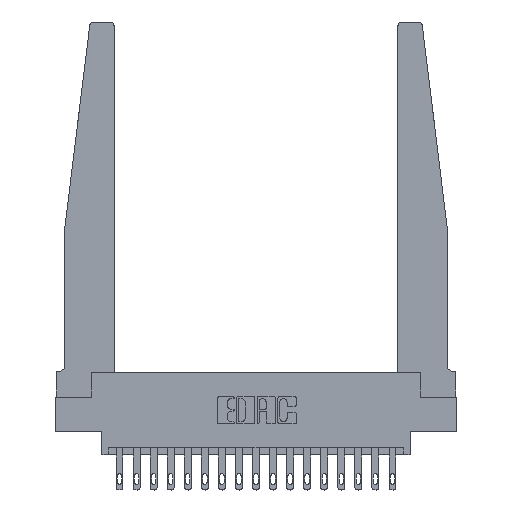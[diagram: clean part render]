
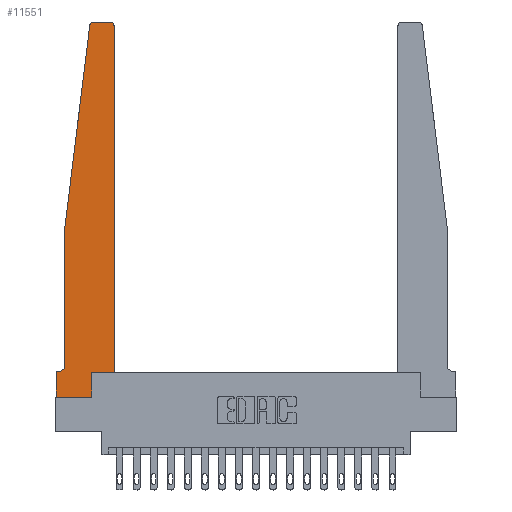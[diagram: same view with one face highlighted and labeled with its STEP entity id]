
A CAD part, top view. The second image highlights one B-rep face of the part: STEP entity #11551.
In plain terms, the highlighted planar face has unit normal (0, 0, 1).
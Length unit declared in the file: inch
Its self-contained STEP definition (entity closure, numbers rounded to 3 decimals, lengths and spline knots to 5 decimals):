
#142 = CARTESIAN_POINT ( 'NONE',  ( 0.425, 0.18, 0.37 ) ) ;
#512 = DIRECTION ( 'NONE',  ( 0., 0., 1. ) ) ;
#813 = AXIS2_PLACEMENT_3D ( 'NONE', #14838, #11664, #16329 ) ;
#840 = VECTOR ( 'NONE', #6981, 39.37008 ) ;
#849 = ORIENTED_EDGE ( 'NONE', *, *, #18544, .T. ) ;
#868 = VECTOR ( 'NONE', #9005, 39.37008 ) ;
#875 = CARTESIAN_POINT ( 'NONE',  ( 0., 0., 0.37 ) ) ;
#973 = CARTESIAN_POINT ( 'NONE',  ( 0.015, 0.2375, 0.37 ) ) ;
#1383 = ORIENTED_EDGE ( 'NONE', *, *, #11961, .T. ) ;
#1763 = VECTOR ( 'NONE', #14503, 39.37008 ) ;
#1956 = CARTESIAN_POINT ( 'NONE',  ( 0.065, 0.2375, 0.37 ) ) ;
#2150 = EDGE_CURVE ( 'NONE', #18866, #17436, #12518, .T. ) ;
#2842 = LINE ( 'NONE', #142, #8823 ) ;
#2949 = ORIENTED_EDGE ( 'NONE', *, *, #14845, .T. ) ;
#3259 = VECTOR ( 'NONE', #5181, 39.37008 ) ;
#3283 = VERTEX_POINT ( 'NONE', #7227 ) ;
#3580 = DIRECTION ( 'NONE',  ( -1., 0., 0. ) ) ;
#3769 = CIRCLE ( 'NONE', #6992, 0.05 ) ;
#3858 = LINE ( 'NONE', #875, #840 ) ;
#3860 = DIRECTION ( 'NONE',  ( 0., -1., 0. ) ) ;
#3970 = VECTOR ( 'NONE', #3860, 39.37008 ) ;
#3993 = EDGE_CURVE ( 'NONE', #12755, #3283, #17140, .T. ) ;
#4364 = VERTEX_POINT ( 'NONE', #14314 ) ;
#4394 = VERTEX_POINT ( 'NONE', #17504 ) ;
#4511 = CARTESIAN_POINT ( 'NONE',  ( 0.2605, 0.18, 0.37 ) ) ;
#4976 = LINE ( 'NONE', #9862, #17024 ) ;
#5012 = CARTESIAN_POINT ( 'NONE',  ( 0., 0.1875, 0.37 ) ) ;
#5181 = DIRECTION ( 'NONE',  ( -1., 0., 0. ) ) ;
#5279 = CIRCLE ( 'NONE', #813, 0.03 ) ;
#5324 = LINE ( 'NONE', #12832, #1763 ) ;
#5334 = AXIS2_PLACEMENT_3D ( 'NONE', #7943, #6639, #14203 ) ;
#5372 = LINE ( 'NONE', #11483, #3970 ) ;
#6398 = VECTOR ( 'NONE', #7916, 39.37008 ) ;
#6484 = ORIENTED_EDGE ( 'NONE', *, *, #13730, .T. ) ;
#6507 = ORIENTED_EDGE ( 'NONE', *, *, #13590, .T. ) ;
#6639 = DIRECTION ( 'NONE',  ( 0., 0., 1. ) ) ;
#6855 = VECTOR ( 'NONE', #16029, 39.37008 ) ;
#6981 = DIRECTION ( 'NONE',  ( 0., -1., 0. ) ) ;
#6992 = AXIS2_PLACEMENT_3D ( 'NONE', #973, #11200, #3580 ) ;
#6995 = CARTESIAN_POINT ( 'NONE',  ( 0.425, 0.18, 0.37 ) ) ;
#7227 = CARTESIAN_POINT ( 'NONE',  ( 0.27653, 2.75, 0.37 ) ) ;
#7452 = CARTESIAN_POINT ( 'NONE',  ( 0.2605, 0., 0.37 ) ) ;
#7617 = ORIENTED_EDGE ( 'NONE', *, *, #2150, .T. ) ;
#7916 = DIRECTION ( 'NONE',  ( 0., 1., 0. ) ) ;
#7943 = CARTESIAN_POINT ( 'NONE',  ( 0.27653, 2.72, 0.37 ) ) ;
#8084 = DIRECTION ( 'NONE',  ( 1., 0., 0. ) ) ;
#8559 = VERTEX_POINT ( 'NONE', #5012 ) ;
#8823 = VECTOR ( 'NONE', #16498, 39.37008 ) ;
#9005 = DIRECTION ( 'NONE',  ( -0.122, -0.992, 0. ) ) ;
#9197 = VERTEX_POINT ( 'NONE', #6995 ) ;
#9204 = CARTESIAN_POINT ( 'NONE',  ( 0.425, 2.72, 0.37 ) ) ;
#9537 = EDGE_LOOP ( 'NONE', ( #12274, #9996, #849, #6484, #1383, #16868, #16133, #2949, #7617, #6507, #15865, #16618 ) ) ;
#9605 = VERTEX_POINT ( 'NONE', #1956 ) ;
#9862 = CARTESIAN_POINT ( 'NONE',  ( 0.425, 0.18, 0.37 ) ) ;
#9996 = ORIENTED_EDGE ( 'NONE', *, *, #18228, .T. ) ;
#10084 = CARTESIAN_POINT ( 'NONE',  ( 0.015, 0.1875, 0.37 ) ) ;
#11200 = DIRECTION ( 'NONE',  ( 0., 0., -1. ) ) ;
#11419 = FACE_OUTER_BOUND ( 'NONE', #9537, .T. ) ;
#11473 = CARTESIAN_POINT ( 'NONE',  ( 0., 0., 0.37 ) ) ;
#11483 = CARTESIAN_POINT ( 'NONE',  ( 0.065, 1.25, 0.37 ) ) ;
#11551 = ADVANCED_FACE ( 'NONE', ( #11419 ), #18980, .T. ) ;
#11660 = LINE ( 'NONE', #11473, #6855 ) ;
#11664 = DIRECTION ( 'NONE',  ( 0., 0., 1. ) ) ;
#11961 = EDGE_CURVE ( 'NONE', #9605, #14570, #3769, .T. ) ;
#12274 = ORIENTED_EDGE ( 'NONE', *, *, #3993, .T. ) ;
#12518 = LINE ( 'NONE', #4511, #6398 ) ;
#12594 = CARTESIAN_POINT ( 'NONE',  ( 0.25, 2.75, 0.37 ) ) ;
#12755 = VERTEX_POINT ( 'NONE', #16577 ) ;
#12832 = CARTESIAN_POINT ( 'NONE',  ( 0.065, 0.1875, 0.37 ) ) ;
#13590 = EDGE_CURVE ( 'NONE', #17436, #9197, #4976, .T. ) ;
#13730 = EDGE_CURVE ( 'NONE', #4364, #9605, #5372, .T. ) ;
#14032 = EDGE_CURVE ( 'NONE', #14570, #8559, #5324, .T. ) ;
#14203 = DIRECTION ( 'NONE',  ( 1., 0., 0. ) ) ;
#14295 = VERTEX_POINT ( 'NONE', #9204 ) ;
#14314 = CARTESIAN_POINT ( 'NONE',  ( 0.065, 1.25, 0.37 ) ) ;
#14394 = CARTESIAN_POINT ( 'NONE',  ( 0., 0.1875, 0.37 ) ) ;
#14503 = DIRECTION ( 'NONE',  ( -1., 0., 0. ) ) ;
#14570 = VERTEX_POINT ( 'NONE', #10084 ) ;
#14838 = CARTESIAN_POINT ( 'NONE',  ( 0.395, 2.72, 0.37 ) ) ;
#14845 = EDGE_CURVE ( 'NONE', #15749, #18866, #11660, .T. ) ;
#15749 = VERTEX_POINT ( 'NONE', #16350 ) ;
#15865 = ORIENTED_EDGE ( 'NONE', *, *, #18075, .T. ) ;
#16029 = DIRECTION ( 'NONE',  ( 1., 0., 0. ) ) ;
#16133 = ORIENTED_EDGE ( 'NONE', *, *, #17519, .T. ) ;
#16172 = EDGE_CURVE ( 'NONE', #14295, #12755, #5279, .T. ) ;
#16329 = DIRECTION ( 'NONE',  ( 1., 0., 0. ) ) ;
#16350 = CARTESIAN_POINT ( 'NONE',  ( 0., 0., 0.37 ) ) ;
#16476 = CARTESIAN_POINT ( 'NONE',  ( 0.065, 1.25, 0.37 ) ) ;
#16498 = DIRECTION ( 'NONE',  ( 0., 1., 0. ) ) ;
#16577 = CARTESIAN_POINT ( 'NONE',  ( 0.395, 2.75, 0.37 ) ) ;
#16618 = ORIENTED_EDGE ( 'NONE', *, *, #16172, .T. ) ;
#16868 = ORIENTED_EDGE ( 'NONE', *, *, #14032, .T. ) ;
#17024 = VECTOR ( 'NONE', #8084, 39.37008 ) ;
#17140 = LINE ( 'NONE', #12594, #3259 ) ;
#17436 = VERTEX_POINT ( 'NONE', #19042 ) ;
#17504 = CARTESIAN_POINT ( 'NONE',  ( 0.24675, 2.72367, 0.37 ) ) ;
#17519 = EDGE_CURVE ( 'NONE', #8559, #15749, #3858, .T. ) ;
#18075 = EDGE_CURVE ( 'NONE', #9197, #14295, #2842, .T. ) ;
#18086 = CIRCLE ( 'NONE', #5334, 0.03 ) ;
#18228 = EDGE_CURVE ( 'NONE', #3283, #4394, #18086, .T. ) ;
#18292 = LINE ( 'NONE', #16476, #868 ) ;
#18544 = EDGE_CURVE ( 'NONE', #4394, #4364, #18292, .T. ) ;
#18866 = VERTEX_POINT ( 'NONE', #7452 ) ;
#18883 = DIRECTION ( 'NONE',  ( 1., 0., 0. ) ) ;
#18980 = PLANE ( 'NONE',  #19664 ) ;
#19042 = CARTESIAN_POINT ( 'NONE',  ( 0.2605, 0.18, 0.37 ) ) ;
#19664 = AXIS2_PLACEMENT_3D ( 'NONE', #14394, #512, #18883 ) ;
